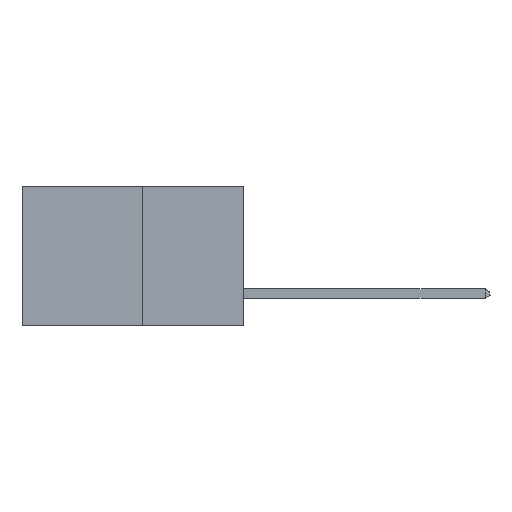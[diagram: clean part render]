
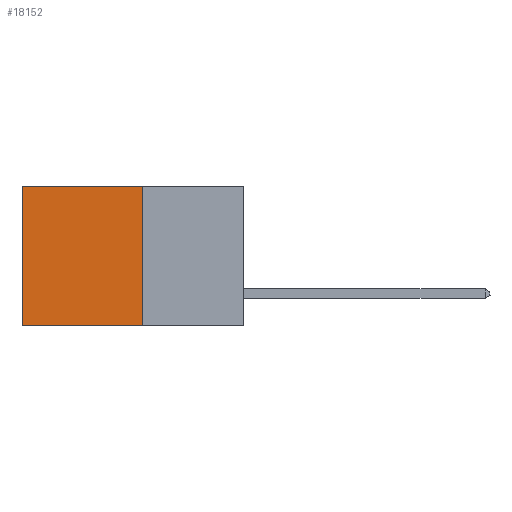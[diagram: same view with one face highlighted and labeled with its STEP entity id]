
A CAD part, left-side view. The second image highlights one B-rep face of the part: STEP entity #18152.
In plain terms, the highlighted planar face has unit normal (-1, 0, 0).
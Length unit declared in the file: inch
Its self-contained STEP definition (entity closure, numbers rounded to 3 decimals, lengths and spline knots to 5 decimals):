
#76 = CARTESIAN_POINT ( 'NONE',  ( 0.277, 0.27, -0.37 ) ) ;
#1248 = AXIS2_PLACEMENT_3D ( 'NONE', #6339, #4910, #15099 ) ;
#1284 = VECTOR ( 'NONE', #12362, 39.37008 ) ;
#2309 = VERTEX_POINT ( 'NONE', #8052 ) ;
#2763 = VERTEX_POINT ( 'NONE', #5461 ) ;
#3260 = EDGE_CURVE ( 'NONE', #2763, #15260, #6999, .T. ) ;
#3368 = PLANE ( 'NONE',  #1248 ) ;
#3594 = CARTESIAN_POINT ( 'NONE',  ( 0.277, 0.27, -0.37 ) ) ;
#4607 = DIRECTION ( 'NONE',  ( 0., 0., -1. ) ) ;
#4711 = EDGE_LOOP ( 'NONE', ( #8734, #13513, #18176, #17035 ) ) ;
#4910 = DIRECTION ( 'NONE',  ( 1., 0., 0. ) ) ;
#5334 = LINE ( 'NONE', #3594, #1284 ) ;
#5461 = CARTESIAN_POINT ( 'NONE',  ( 0.277, 0.27, 0. ) ) ;
#5982 = LINE ( 'NONE', #11844, #9356 ) ;
#6339 = CARTESIAN_POINT ( 'NONE',  ( 0.277, 0.27, -0.37 ) ) ;
#6999 = LINE ( 'NONE', #15527, #14283 ) ;
#7450 = CARTESIAN_POINT ( 'NONE',  ( 0.277, 0.59, 0. ) ) ;
#8052 = CARTESIAN_POINT ( 'NONE',  ( 0.277, 0.59, -0.37 ) ) ;
#8734 = ORIENTED_EDGE ( 'NONE', *, *, #17224, .T. ) ;
#9356 = VECTOR ( 'NONE', #4607, 39.37008 ) ;
#11614 = EDGE_CURVE ( 'NONE', #15944, #2309, #5334, .T. ) ;
#11844 = CARTESIAN_POINT ( 'NONE',  ( 0.277, 0.59, -0.37 ) ) ;
#11850 = LINE ( 'NONE', #14904, #12308 ) ;
#12308 = VECTOR ( 'NONE', #14965, 39.37008 ) ;
#12316 = EDGE_CURVE ( 'NONE', #2763, #15944, #11850, .T. ) ;
#12362 = DIRECTION ( 'NONE',  ( 0., 1., 0. ) ) ;
#13513 = ORIENTED_EDGE ( 'NONE', *, *, #11614, .F. ) ;
#14283 = VECTOR ( 'NONE', #15585, 39.37008 ) ;
#14904 = CARTESIAN_POINT ( 'NONE',  ( 0.277, 0.27, -0.37 ) ) ;
#14965 = DIRECTION ( 'NONE',  ( 0., 0., -1. ) ) ;
#15099 = DIRECTION ( 'NONE',  ( 0., 0., -1. ) ) ;
#15260 = VERTEX_POINT ( 'NONE', #7450 ) ;
#15527 = CARTESIAN_POINT ( 'NONE',  ( 0.277, 0.27, 0. ) ) ;
#15585 = DIRECTION ( 'NONE',  ( 0., 1., 0. ) ) ;
#15670 = FACE_OUTER_BOUND ( 'NONE', #4711, .T. ) ;
#15944 = VERTEX_POINT ( 'NONE', #76 ) ;
#17035 = ORIENTED_EDGE ( 'NONE', *, *, #3260, .T. ) ;
#17224 = EDGE_CURVE ( 'NONE', #15260, #2309, #5982, .T. ) ;
#18152 = ADVANCED_FACE ( 'NONE', ( #15670 ), #3368, .F. ) ;
#18176 = ORIENTED_EDGE ( 'NONE', *, *, #12316, .F. ) ;
